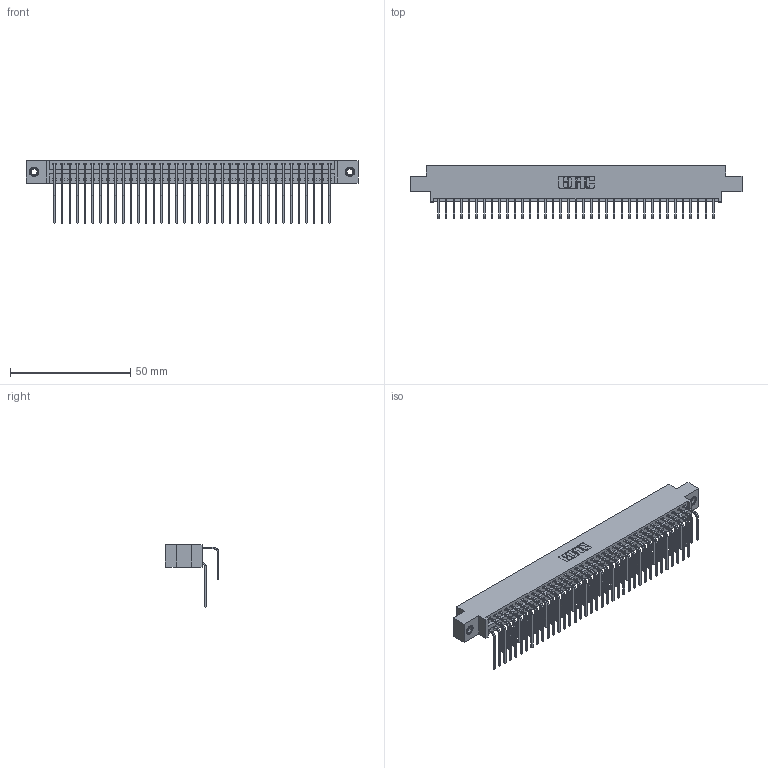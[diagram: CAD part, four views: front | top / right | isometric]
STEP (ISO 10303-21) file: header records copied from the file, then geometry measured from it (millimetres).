
FILE_DESCRIPTION (( 'STEP AP203' ), '1' );
FILE_NAME ('346-074-558-807.STEP', '2022-05-25T03:32:37', ( '' ), ( '' ), 'SwSTEP 2.0', 'SolidWorks 2020', '' );
FILE_SCHEMA (( 'CONFIG_CONTROL_DESIGN' ));
Length unit declared in the file: inch
Products named in the file (5): 346 Part_0.170 Offset - 0.156 Dia-TI; 345-292-001_558 Tail - 2; 345-292-001_558 559 Tail - 1; 345-250-001_345-250-005-103; 346-074-558-807
Assembly tree (77 placements, depth 2):
  346-074-558-807
    346 Part_0.170 Offset - 0.156 Dia-TI
    345-292-001_558 559 Tail - 1  x37
    345-292-001_558 Tail - 2  x37
    345-250-001_345-250-005-103  x2
Bounding box: 138.05 x 22.16 x 26.16 mm (x, y, z)
Volume: 13681.4 mm3; surface area: 20988.7 mm2
Topology: 77 solids, 77 shells, 4182 faces, 12391 edges, 8154 vertices
Faces by surface type: plane 2850, cylinder 1316, cone 12, torus 4
Entity records: 27922 total; most frequent: CARTESIAN_POINT 4646, ORIENTED_EDGE 4522, DIRECTION 4143, EDGE_CURVE 2261, LINE 1921, VECTOR 1921, VERTEX_POINT 1500, AXIS2_PLACEMENT_3D 1111
